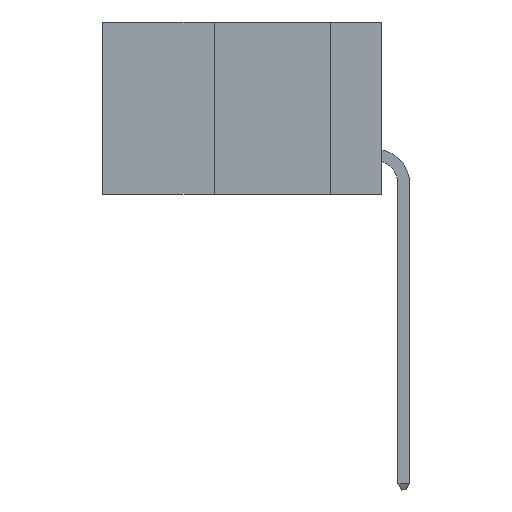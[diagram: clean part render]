
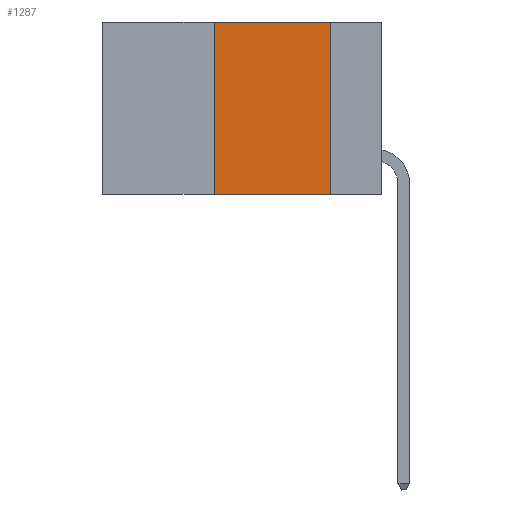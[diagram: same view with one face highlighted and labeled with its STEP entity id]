
A CAD part, left-side view. The second image highlights one B-rep face of the part: STEP entity #1287.
In plain terms, the highlighted planar face has unit normal (-1, 0, 0).
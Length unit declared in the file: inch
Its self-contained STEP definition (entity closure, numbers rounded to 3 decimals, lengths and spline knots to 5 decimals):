
#246 = VECTOR ( 'NONE', #9079, 39.37008 ) ;
#408 = VECTOR ( 'NONE', #3734, 39.37008 ) ;
#856 = DIRECTION ( 'NONE',  ( 0., 0., -1. ) ) ;
#1287 = ADVANCED_FACE ( 'NONE', ( #8201 ), #1484, .F. ) ;
#1338 = LINE ( 'NONE', #11164, #11940 ) ;
#1484 = PLANE ( 'NONE',  #15939 ) ;
#1551 = VERTEX_POINT ( 'NONE', #6647 ) ;
#1851 = ORIENTED_EDGE ( 'NONE', *, *, #11624, .F. ) ;
#2630 = CARTESIAN_POINT ( 'NONE',  ( 0., 0.6, 0. ) ) ;
#2863 = VERTEX_POINT ( 'NONE', #5636 ) ;
#3725 = EDGE_LOOP ( 'NONE', ( #15892, #16341, #1851, #7445 ) ) ;
#3734 = DIRECTION ( 'NONE',  ( 0., -1., 0. ) ) ;
#4243 = CARTESIAN_POINT ( 'NONE',  ( 0., 0.36, 0. ) ) ;
#4593 = LINE ( 'NONE', #4243, #11566 ) ;
#5109 = CARTESIAN_POINT ( 'NONE',  ( 0., 0.6, 0. ) ) ;
#5227 = EDGE_CURVE ( 'NONE', #8455, #12538, #1338, .T. ) ;
#5305 = DIRECTION ( 'NONE',  ( 1., 0., 0. ) ) ;
#5636 = CARTESIAN_POINT ( 'NONE',  ( 0., 0.36, -0.37 ) ) ;
#6023 = CARTESIAN_POINT ( 'NONE',  ( 0., 0.11, 0. ) ) ;
#6583 = DIRECTION ( 'NONE',  ( 0., 0., -1. ) ) ;
#6647 = CARTESIAN_POINT ( 'NONE',  ( 0., 0.36, 0. ) ) ;
#7361 = LINE ( 'NONE', #12904, #408 ) ;
#7427 = LINE ( 'NONE', #5109, #246 ) ;
#7445 = ORIENTED_EDGE ( 'NONE', *, *, #16143, .T. ) ;
#8201 = FACE_OUTER_BOUND ( 'NONE', #3725, .T. ) ;
#8455 = VERTEX_POINT ( 'NONE', #6023 ) ;
#8589 = CARTESIAN_POINT ( 'NONE',  ( 0., 0.11, -0.37 ) ) ;
#9079 = DIRECTION ( 'NONE',  ( 0., -1., 0. ) ) ;
#11164 = CARTESIAN_POINT ( 'NONE',  ( 0., 0.11, 0. ) ) ;
#11566 = VECTOR ( 'NONE', #16206, 39.37008 ) ;
#11624 = EDGE_CURVE ( 'NONE', #2863, #1551, #4593, .T. ) ;
#11940 = VECTOR ( 'NONE', #856, 39.37008 ) ;
#12538 = VERTEX_POINT ( 'NONE', #8589 ) ;
#12904 = CARTESIAN_POINT ( 'NONE',  ( 0., 0.6, -0.37 ) ) ;
#14691 = EDGE_CURVE ( 'NONE', #1551, #8455, #7427, .T. ) ;
#15892 = ORIENTED_EDGE ( 'NONE', *, *, #5227, .F. ) ;
#15939 = AXIS2_PLACEMENT_3D ( 'NONE', #2630, #5305, #6583 ) ;
#16143 = EDGE_CURVE ( 'NONE', #2863, #12538, #7361, .T. ) ;
#16206 = DIRECTION ( 'NONE',  ( 0., 0., 1. ) ) ;
#16341 = ORIENTED_EDGE ( 'NONE', *, *, #14691, .F. ) ;
